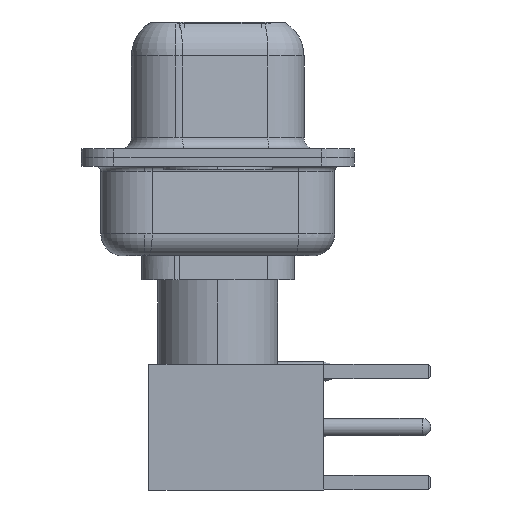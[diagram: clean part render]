
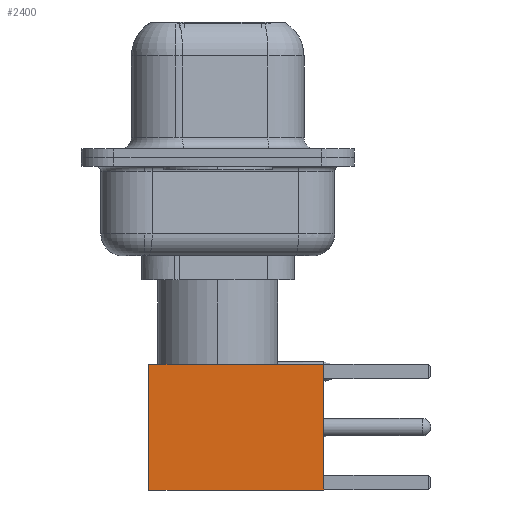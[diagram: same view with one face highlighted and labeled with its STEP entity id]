
A CAD part, left-side view. The second image highlights one B-rep face of the part: STEP entity #2400.
In plain terms, the highlighted face is planar.
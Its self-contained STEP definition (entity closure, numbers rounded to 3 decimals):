
#294 = VECTOR ( 'NONE', #3543, 1000. ) ;
#962 = CARTESIAN_POINT ( 'NONE',  ( 0., 2.875, 0. ) ) ;
#965 = ORIENTED_EDGE ( 'NONE', *, *, #10082, .F. ) ;
#2400 = ADVANCED_FACE ( 'NONE', ( #8122 ), #8377, .T. ) ;
#2447 = EDGE_LOOP ( 'NONE', ( #17657, #12911, #11311, #965 ) ) ;
#2456 = CARTESIAN_POINT ( 'NONE',  ( 2.875, 2.875, 8. ) ) ;
#2651 = EDGE_CURVE ( 'NONE', #3700, #23435, #5547, .T. ) ;
#3543 = DIRECTION ( 'NONE',  ( 0., 0., -1. ) ) ;
#3700 = VERTEX_POINT ( 'NONE', #2456 ) ;
#4503 = VECTOR ( 'NONE', #4705, 1000. ) ;
#4615 = AXIS2_PLACEMENT_3D ( 'NONE', #16516, #16254, #24417 ) ;
#4705 = DIRECTION ( 'NONE',  ( -1., 0., 0. ) ) ;
#4845 = LINE ( 'NONE', #962, #23944 ) ;
#5000 = LINE ( 'NONE', #13921, #16164 ) ;
#5523 = EDGE_CURVE ( 'NONE', #23435, #22814, #4845, .T. ) ;
#5547 = LINE ( 'NONE', #20092, #294 ) ;
#6035 = CARTESIAN_POINT ( 'NONE',  ( 2.875, 2.875, 0. ) ) ;
#7418 = CARTESIAN_POINT ( 'NONE',  ( -2.875, 2.875, 0. ) ) ;
#7695 = VERTEX_POINT ( 'NONE', #25911 ) ;
#8122 = FACE_OUTER_BOUND ( 'NONE', #2447, .T. ) ;
#8377 = PLANE ( 'NONE',  #4615 ) ;
#10082 = EDGE_CURVE ( 'NONE', #3700, #7695, #14734, .T. ) ;
#11311 = ORIENTED_EDGE ( 'NONE', *, *, #21476, .F. ) ;
#11399 = DIRECTION ( 'NONE',  ( -1., 0., 0. ) ) ;
#12911 = ORIENTED_EDGE ( 'NONE', *, *, #5523, .T. ) ;
#13921 = CARTESIAN_POINT ( 'NONE',  ( -2.875, 2.875, 0. ) ) ;
#14734 = LINE ( 'NONE', #15002, #4503 ) ;
#15002 = CARTESIAN_POINT ( 'NONE',  ( 0., 2.875, 8. ) ) ;
#16164 = VECTOR ( 'NONE', #26211, 1000. ) ;
#16254 = DIRECTION ( 'NONE',  ( 0., 1., 0. ) ) ;
#16516 = CARTESIAN_POINT ( 'NONE',  ( 2.875, 2.875, 0. ) ) ;
#17657 = ORIENTED_EDGE ( 'NONE', *, *, #2651, .T. ) ;
#20092 = CARTESIAN_POINT ( 'NONE',  ( 2.875, 2.875, 0. ) ) ;
#21476 = EDGE_CURVE ( 'NONE', #7695, #22814, #5000, .T. ) ;
#22814 = VERTEX_POINT ( 'NONE', #7418 ) ;
#23435 = VERTEX_POINT ( 'NONE', #6035 ) ;
#23944 = VECTOR ( 'NONE', #11399, 1000. ) ;
#24417 = DIRECTION ( 'NONE',  ( 0., 0., 1. ) ) ;
#25911 = CARTESIAN_POINT ( 'NONE',  ( -2.875, 2.875, 8. ) ) ;
#26211 = DIRECTION ( 'NONE',  ( 0., 0., -1. ) ) ;
